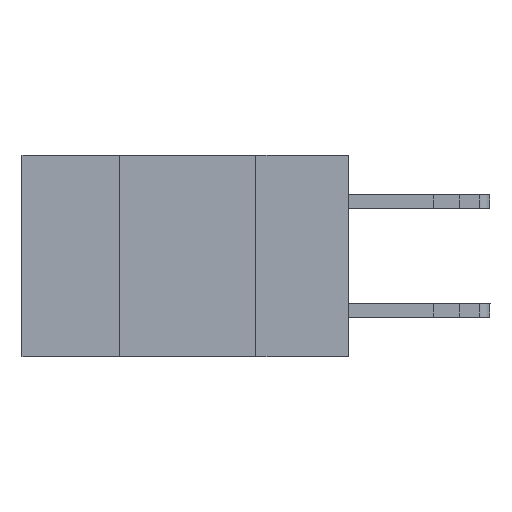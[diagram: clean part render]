
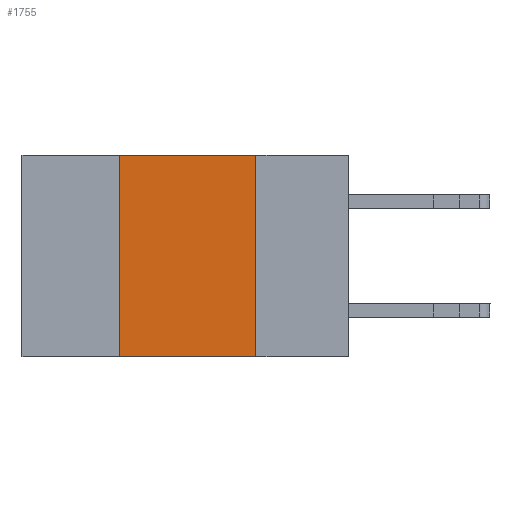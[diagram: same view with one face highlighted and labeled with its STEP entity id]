
A CAD part, left-side view. The second image highlights one B-rep face of the part: STEP entity #1755.
In plain terms, the highlighted planar face has unit normal (-1, 0, 0).
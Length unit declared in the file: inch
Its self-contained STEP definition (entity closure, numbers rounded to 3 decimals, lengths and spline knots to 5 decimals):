
#112 = ORIENTED_EDGE ( 'NONE', *, *, #2060, .F. ) ;
#474 = DIRECTION ( 'NONE',  ( 0., 0., 1. ) ) ;
#1018 = FACE_OUTER_BOUND ( 'NONE', #3691, .T. ) ;
#1088 = EDGE_CURVE ( 'NONE', #6101, #15194, #8430, .T. ) ;
#1755 = ADVANCED_FACE ( 'NONE', ( #1018 ), #12537, .F. ) ;
#1812 = VERTEX_POINT ( 'NONE', #18412 ) ;
#1863 = CARTESIAN_POINT ( 'NONE',  ( 0., 0.42, 0. ) ) ;
#2060 = EDGE_CURVE ( 'NONE', #8054, #6101, #14162, .T. ) ;
#2483 = DIRECTION ( 'NONE',  ( 0., -1., 0. ) ) ;
#3320 = ORIENTED_EDGE ( 'NONE', *, *, #17718, .F. ) ;
#3342 = CARTESIAN_POINT ( 'NONE',  ( 0., 0.42, -0.37 ) ) ;
#3691 = EDGE_LOOP ( 'NONE', ( #3320, #5541, #112, #7743 ) ) ;
#3763 = DIRECTION ( 'NONE',  ( 0., 0., -1. ) ) ;
#4095 = DIRECTION ( 'NONE',  ( 1., 0., 0. ) ) ;
#4401 = VECTOR ( 'NONE', #10044, 39.37008 ) ;
#5296 = LINE ( 'NONE', #17139, #4401 ) ;
#5541 = ORIENTED_EDGE ( 'NONE', *, *, #1088, .F. ) ;
#5684 = AXIS2_PLACEMENT_3D ( 'NONE', #11184, #4095, #14029 ) ;
#6101 = VERTEX_POINT ( 'NONE', #1863 ) ;
#6614 = CARTESIAN_POINT ( 'NONE',  ( 0., 0.17, -0.37 ) ) ;
#7743 = ORIENTED_EDGE ( 'NONE', *, *, #8739, .T. ) ;
#8054 = VERTEX_POINT ( 'NONE', #8613 ) ;
#8085 = CARTESIAN_POINT ( 'NONE',  ( 0., 0.17, 0. ) ) ;
#8430 = LINE ( 'NONE', #13856, #11329 ) ;
#8613 = CARTESIAN_POINT ( 'NONE',  ( 0., 0.42, -0.37 ) ) ;
#8739 = EDGE_CURVE ( 'NONE', #8054, #1812, #5296, .T. ) ;
#10044 = DIRECTION ( 'NONE',  ( 0., -1., 0. ) ) ;
#11184 = CARTESIAN_POINT ( 'NONE',  ( 0., 0.6, 0. ) ) ;
#11314 = LINE ( 'NONE', #6614, #18021 ) ;
#11329 = VECTOR ( 'NONE', #2483, 39.37008 ) ;
#12537 = PLANE ( 'NONE',  #5684 ) ;
#13720 = VECTOR ( 'NONE', #474, 39.37008 ) ;
#13856 = CARTESIAN_POINT ( 'NONE',  ( 0., 0.6, 0. ) ) ;
#14029 = DIRECTION ( 'NONE',  ( 0., 0., -1. ) ) ;
#14162 = LINE ( 'NONE', #3342, #13720 ) ;
#15194 = VERTEX_POINT ( 'NONE', #8085 ) ;
#17139 = CARTESIAN_POINT ( 'NONE',  ( 0., 0.6, -0.37 ) ) ;
#17718 = EDGE_CURVE ( 'NONE', #15194, #1812, #11314, .T. ) ;
#18021 = VECTOR ( 'NONE', #3763, 39.37008 ) ;
#18412 = CARTESIAN_POINT ( 'NONE',  ( 0., 0.17, -0.37 ) ) ;
